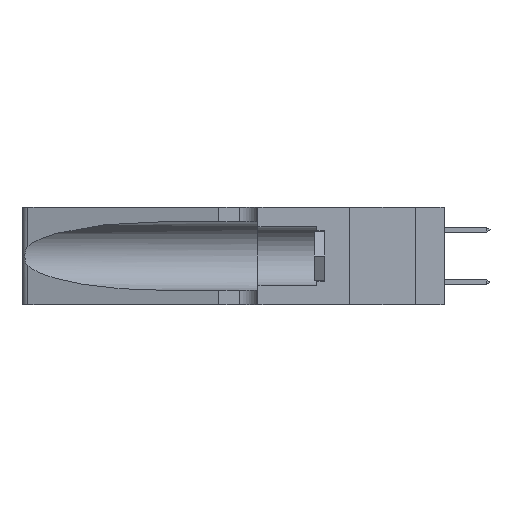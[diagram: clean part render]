
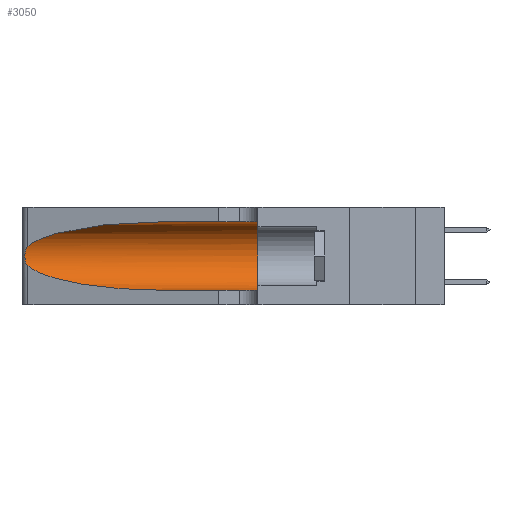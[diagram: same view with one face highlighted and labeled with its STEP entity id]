
A CAD part, left-side view. The second image highlights one B-rep face of the part: STEP entity #3050.
In plain terms, the highlighted cylindrical face has radius 3.308 mm (diameter 6.617 mm), a partial arc.
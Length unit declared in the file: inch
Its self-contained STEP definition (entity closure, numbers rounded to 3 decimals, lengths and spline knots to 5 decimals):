
#5 = CARTESIAN_POINT ( 'NONE',  ( 0.2373, 1.15595, 0.28018 ) ) ;
#175 = CARTESIAN_POINT ( 'NONE',  ( 0.1305, 0.35, 0.185 ) ) ;
#250 = DIRECTION ( 'NONE',  ( 0., 0., 1. ) ) ;
#1095 = CARTESIAN_POINT ( 'NONE',  ( 0.18966, 0.96281, 0.05475 ) ) ;
#1317 = CARTESIAN_POINT ( 'NONE',  ( 0.25487, 1.22718, 0.14631 ) ) ;
#1714 = CARTESIAN_POINT ( 'NONE',  ( 0.25555, 1.22993, 0.14849 ) ) ;
#1742 = B_SPLINE_CURVE_WITH_KNOTS ( 'NONE', 3,
 ( #8706, #5474, #14006, #15707, #12227, #8904, #4037, #15506, #3013, #20656, #10993, #14294, #1714, #14782 ),
 .UNSPECIFIED., .F., .F.,
 ( 4, 2, 2, 2, 2, 2, 4 ),
 ( 0., 0.00027, 0.00053, 0.00107, 0.0016, 0.00187, 0.00214 ),
 .UNSPECIFIED. ) ;
#1794 = EDGE_CURVE ( 'NONE', #15672, #19341, #17441, .T. ) ;
#2366 = VECTOR ( 'NONE', #4194, 39.37008 ) ;
#2486 = EDGE_CURVE ( 'NONE', #15702, #11603, #6157, .T. ) ;
#2666 = CARTESIAN_POINT ( 'NONE',  ( 0.2373, 1.15595, 0.08982 ) ) ;
#2748 = ORIENTED_EDGE ( 'NONE', *, *, #8673, .F. ) ;
#2858 = CYLINDRICAL_SURFACE ( 'NONE', #18625, 0.13025 ) ;
#3013 = CARTESIAN_POINT ( 'NONE',  ( 0.26017, 1.23833, 0.17102 ) ) ;
#3050 = ADVANCED_FACE ( 'NONE', ( #11280 ), #2858, .F. ) ;
#3755 = VERTEX_POINT ( 'NONE', #10313 ) ;
#3786 = EDGE_LOOP ( 'NONE', ( #8316, #4863, #19523, #14705, #18652, #2748 ) ) ;
#4037 = CARTESIAN_POINT ( 'NONE',  ( 0.26075, 1.23896, 0.19203 ) ) ;
#4194 = DIRECTION ( 'NONE',  ( 0., -1., 0. ) ) ;
#4251 = CARTESIAN_POINT ( 'NONE',  ( 0.1305, 1.61858, 0.31525 ) ) ;
#4383 = CARTESIAN_POINT ( 'NONE',  ( 0.1305, 0.72297, 0.05475 ) ) ;
#4863 = ORIENTED_EDGE ( 'NONE', *, *, #5554, .T. ) ;
#5474 = CARTESIAN_POINT ( 'NONE',  ( 0.25555, 1.22994, 0.2215 ) ) ;
#5554 = EDGE_CURVE ( 'NONE', #3755, #15702, #1742, .T. ) ;
#6029 = AXIS2_PLACEMENT_3D ( 'NONE', #175, #6842, #250 ) ;
#6117 = CARTESIAN_POINT ( 'NONE',  ( 0.1305, 1.61858, 0.185 ) ) ;
#6157 =( BOUNDED_CURVE ( )  B_SPLINE_CURVE ( 3, ( #1317, #2666, #1095, #4383 ),
 .UNSPECIFIED., .F., .F. ) 
 B_SPLINE_CURVE_WITH_KNOTS ( ( 4, 4 ),
 ( 3.44316, 4.71239 ),
 .UNSPECIFIED. ) 
 CURVE ( )  GEOMETRIC_REPRESENTATION_ITEM ( )  RATIONAL_B_SPLINE_CURVE ( ( 1., 0.87, 0.87, 1. ) ) 
 REPRESENTATION_ITEM ( '' )  );
#6192 = EDGE_CURVE ( 'NONE', #13928, #3755, #14448, .T. ) ;
#6842 = DIRECTION ( 'NONE',  ( 0., 1., 0. ) ) ;
#7506 = CARTESIAN_POINT ( 'NONE',  ( 0.1305, 0.35, 0.05475 ) ) ;
#8119 = CARTESIAN_POINT ( 'NONE',  ( 0.25487, 1.22718, 0.14631 ) ) ;
#8316 = ORIENTED_EDGE ( 'NONE', *, *, #6192, .T. ) ;
#8673 = EDGE_CURVE ( 'NONE', #13928, #15672, #16646, .T. ) ;
#8706 = CARTESIAN_POINT ( 'NONE',  ( 0.25487, 1.22718, 0.22369 ) ) ;
#8904 = CARTESIAN_POINT ( 'NONE',  ( 0.26018, 1.23835, 0.19895 ) ) ;
#9066 = DIRECTION ( 'NONE',  ( 0., -1., 0. ) ) ;
#9255 = CARTESIAN_POINT ( 'NONE',  ( 0.1305, 0.72297, 0.05475 ) ) ;
#9791 = CARTESIAN_POINT ( 'NONE',  ( 0.25487, 1.22718, 0.22369 ) ) ;
#10313 = CARTESIAN_POINT ( 'NONE',  ( 0.25487, 1.22718, 0.22369 ) ) ;
#10993 = CARTESIAN_POINT ( 'NONE',  ( 0.25789, 1.23486, 0.15765 ) ) ;
#11280 = FACE_OUTER_BOUND ( 'NONE', #3786, .T. ) ;
#11603 = VERTEX_POINT ( 'NONE', #9255 ) ;
#11743 = CARTESIAN_POINT ( 'NONE',  ( 0.1305, 0.72297, 0.31525 ) ) ;
#12227 = CARTESIAN_POINT ( 'NONE',  ( 0.25854, 1.2359, 0.20912 ) ) ;
#12402 = CARTESIAN_POINT ( 'NONE',  ( 0.1305, 1.61858, 0.05475 ) ) ;
#13928 = VERTEX_POINT ( 'NONE', #11743 ) ;
#14006 = CARTESIAN_POINT ( 'NONE',  ( 0.25639, 1.23184, 0.21858 ) ) ;
#14294 = CARTESIAN_POINT ( 'NONE',  ( 0.25639, 1.23186, 0.15144 ) ) ;
#14448 =( BOUNDED_CURVE ( )  B_SPLINE_CURVE ( 3, ( #16388, #19367, #5, #9791 ),
 .UNSPECIFIED., .F., .T. ) 
 B_SPLINE_CURVE_WITH_KNOTS ( ( 4, 4 ),
 ( 1.5708, 2.84003 ),
 .UNSPECIFIED. ) 
 CURVE ( )  GEOMETRIC_REPRESENTATION_ITEM ( )  RATIONAL_B_SPLINE_CURVE ( ( 1., 0.87, 0.87, 1. ) ) 
 REPRESENTATION_ITEM ( '' )  );
#14705 = ORIENTED_EDGE ( 'NONE', *, *, #17804, .T. ) ;
#14782 = CARTESIAN_POINT ( 'NONE',  ( 0.25487, 1.22718, 0.14631 ) ) ;
#15506 = CARTESIAN_POINT ( 'NONE',  ( 0.26075, 1.23896, 0.178 ) ) ;
#15672 = VERTEX_POINT ( 'NONE', #18155 ) ;
#15702 = VERTEX_POINT ( 'NONE', #8119 ) ;
#15707 = CARTESIAN_POINT ( 'NONE',  ( 0.25787, 1.23484, 0.2124 ) ) ;
#15891 = VECTOR ( 'NONE', #9066, 39.37008 ) ;
#16075 = DIRECTION ( 'NONE',  ( 0., 0., -1. ) ) ;
#16388 = CARTESIAN_POINT ( 'NONE',  ( 0.1305, 0.72297, 0.31525 ) ) ;
#16646 = LINE ( 'NONE', #4251, #15891 ) ;
#17400 = LINE ( 'NONE', #12402, #2366 ) ;
#17441 = CIRCLE ( 'NONE', #6029, 0.13025 ) ;
#17543 = DIRECTION ( 'NONE',  ( 0., -1., 0. ) ) ;
#17804 = EDGE_CURVE ( 'NONE', #11603, #19341, #17400, .T. ) ;
#18155 = CARTESIAN_POINT ( 'NONE',  ( 0.1305, 0.35, 0.31525 ) ) ;
#18625 = AXIS2_PLACEMENT_3D ( 'NONE', #6117, #17543, #16075 ) ;
#18652 = ORIENTED_EDGE ( 'NONE', *, *, #1794, .F. ) ;
#19341 = VERTEX_POINT ( 'NONE', #7506 ) ;
#19367 = CARTESIAN_POINT ( 'NONE',  ( 0.18966, 0.96281, 0.31525 ) ) ;
#19523 = ORIENTED_EDGE ( 'NONE', *, *, #2486, .T. ) ;
#20656 = CARTESIAN_POINT ( 'NONE',  ( 0.25856, 1.23593, 0.16098 ) ) ;
